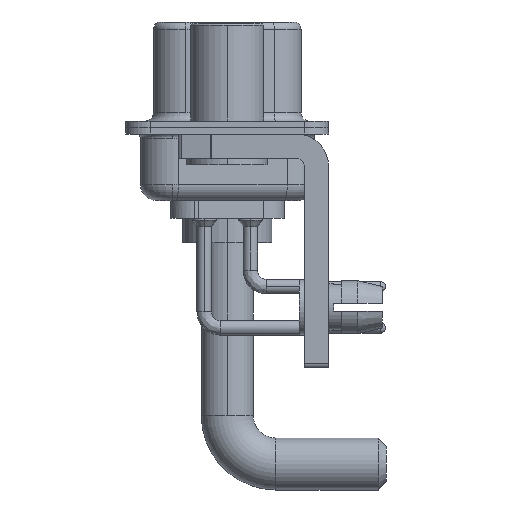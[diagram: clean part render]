
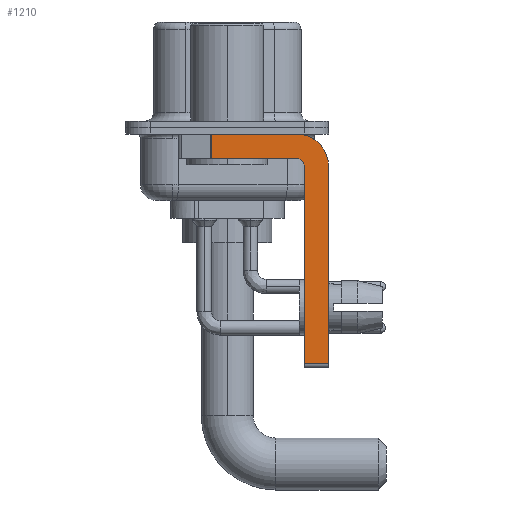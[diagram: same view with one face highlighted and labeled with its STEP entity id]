
A CAD part, left-side view. The second image highlights one B-rep face of the part: STEP entity #1210.
In plain terms, the highlighted planar face has unit normal (-1, 0, 0).
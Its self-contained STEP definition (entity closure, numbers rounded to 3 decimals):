
#480 = EDGE_LOOP ( 'NONE', ( #19807, #501, #16413, #14177, #4503, #20242, #6594, #23680 ) ) ;
#501 = ORIENTED_EDGE ( 'NONE', *, *, #6013, .T. ) ;
#781 = CARTESIAN_POINT ( 'NONE',  ( -2.9, -4.25, -0.4 ) ) ;
#921 = VERTEX_POINT ( 'NONE', #22389 ) ;
#944 = DIRECTION ( 'NONE',  ( 0., 0., -1. ) ) ;
#1027 = LINE ( 'NONE', #12141, #16594 ) ;
#1210 = ADVANCED_FACE ( 'NONE', ( #3372 ), #12655, .F. ) ;
#1835 = CARTESIAN_POINT ( 'NONE',  ( -2.9, -4.25, -2.4 ) ) ;
#1928 = DIRECTION ( 'NONE',  ( 0., -1., 0. ) ) ;
#2697 = DIRECTION ( 'NONE',  ( 0., 0., 1. ) ) ;
#3012 = CARTESIAN_POINT ( 'NONE',  ( -2.9, -4.25, -2.4 ) ) ;
#3253 = VERTEX_POINT ( 'NONE', #24991 ) ;
#3372 = FACE_OUTER_BOUND ( 'NONE', #480, .T. ) ;
#3839 = CARTESIAN_POINT ( 'NONE',  ( -2.9, -6.25, -2.4 ) ) ;
#4288 = CIRCLE ( 'NONE', #28021, 2. ) ;
#4343 = CARTESIAN_POINT ( 'NONE',  ( -2.9, -4.25, -14.55 ) ) ;
#4503 = ORIENTED_EDGE ( 'NONE', *, *, #25401, .F. ) ;
#4635 = LINE ( 'NONE', #4343, #18457 ) ;
#5493 = DIRECTION ( 'NONE',  ( 1., 0., 0. ) ) ;
#5538 = LINE ( 'NONE', #7837, #13043 ) ;
#5593 = VERTEX_POINT ( 'NONE', #27195 ) ;
#5756 = VECTOR ( 'NONE', #2697, 1000. ) ;
#6013 = EDGE_CURVE ( 'NONE', #3253, #921, #9756, .T. ) ;
#6594 = ORIENTED_EDGE ( 'NONE', *, *, #28598, .F. ) ;
#6961 = LINE ( 'NONE', #25174, #5756 ) ;
#7043 = VECTOR ( 'NONE', #12027, 1000. ) ;
#7492 = VERTEX_POINT ( 'NONE', #781 ) ;
#7837 = CARTESIAN_POINT ( 'NONE',  ( -2.9, 3., -0.4 ) ) ;
#8953 = CARTESIAN_POINT ( 'NONE',  ( -2.9, -4.25, -1.9 ) ) ;
#9756 = LINE ( 'NONE', #14622, #7043 ) ;
#11000 = CARTESIAN_POINT ( 'NONE',  ( -2.9, -4.75, -14.55 ) ) ;
#12027 = DIRECTION ( 'NONE',  ( 0., 0., -1. ) ) ;
#12141 = CARTESIAN_POINT ( 'NONE',  ( -2.9, -6.25, -2.4 ) ) ;
#12408 = CARTESIAN_POINT ( 'NONE',  ( -2.9, -4.25, -1.9 ) ) ;
#12599 = DIRECTION ( 'NONE',  ( -1., 0., 0. ) ) ;
#12655 = PLANE ( 'NONE',  #13497 ) ;
#12913 = VERTEX_POINT ( 'NONE', #11000 ) ;
#12959 = DIRECTION ( 'NONE',  ( 0., 0., -1. ) ) ;
#13043 = VECTOR ( 'NONE', #17099, 1000. ) ;
#13497 = AXIS2_PLACEMENT_3D ( 'NONE', #1835, #29456, #12959 ) ;
#14177 = ORIENTED_EDGE ( 'NONE', *, *, #24226, .F. ) ;
#14622 = CARTESIAN_POINT ( 'NONE',  ( -2.9, 0.978, -1.9 ) ) ;
#15515 = DIRECTION ( 'NONE',  ( 0., 1., 0. ) ) ;
#16413 = ORIENTED_EDGE ( 'NONE', *, *, #25262, .F. ) ;
#16594 = VECTOR ( 'NONE', #21378, 1000. ) ;
#16949 = AXIS2_PLACEMENT_3D ( 'NONE', #3012, #12599, #26365 ) ;
#17099 = DIRECTION ( 'NONE',  ( 0., -1., 0. ) ) ;
#18457 = VECTOR ( 'NONE', #1928, 1000. ) ;
#19239 = VERTEX_POINT ( 'NONE', #12408 ) ;
#19807 = ORIENTED_EDGE ( 'NONE', *, *, #24771, .F. ) ;
#20242 = ORIENTED_EDGE ( 'NONE', *, *, #27013, .T. ) ;
#20532 = VERTEX_POINT ( 'NONE', #24381 ) ;
#21378 = DIRECTION ( 'NONE',  ( 0., 0., -1. ) ) ;
#22046 = CARTESIAN_POINT ( 'NONE',  ( -2.9, -4.25, -2.4 ) ) ;
#22176 = LINE ( 'NONE', #8953, #26571 ) ;
#22389 = CARTESIAN_POINT ( 'NONE',  ( -2.9, 0.978, -1.9 ) ) ;
#23332 = EDGE_CURVE ( 'NONE', #7492, #23453, #4288, .T. ) ;
#23453 = VERTEX_POINT ( 'NONE', #3839 ) ;
#23680 = ORIENTED_EDGE ( 'NONE', *, *, #23332, .F. ) ;
#24226 = EDGE_CURVE ( 'NONE', #20532, #19239, #24692, .T. ) ;
#24381 = CARTESIAN_POINT ( 'NONE',  ( -2.9, -4.75, -2.4 ) ) ;
#24692 = CIRCLE ( 'NONE', #16949, 0.5 ) ;
#24771 = EDGE_CURVE ( 'NONE', #3253, #7492, #5538, .T. ) ;
#24991 = CARTESIAN_POINT ( 'NONE',  ( -2.9, 0.978, -0.4 ) ) ;
#25174 = CARTESIAN_POINT ( 'NONE',  ( -2.9, -4.75, -14.8 ) ) ;
#25262 = EDGE_CURVE ( 'NONE', #19239, #921, #22176, .T. ) ;
#25401 = EDGE_CURVE ( 'NONE', #12913, #20532, #6961, .T. ) ;
#26365 = DIRECTION ( 'NONE',  ( 0., 0., 1. ) ) ;
#26571 = VECTOR ( 'NONE', #15515, 1000. ) ;
#27013 = EDGE_CURVE ( 'NONE', #12913, #5593, #4635, .T. ) ;
#27195 = CARTESIAN_POINT ( 'NONE',  ( -2.9, -6.25, -14.55 ) ) ;
#28021 = AXIS2_PLACEMENT_3D ( 'NONE', #22046, #5493, #944 ) ;
#28598 = EDGE_CURVE ( 'NONE', #23453, #5593, #1027, .T. ) ;
#29456 = DIRECTION ( 'NONE',  ( 1., 0., 0. ) ) ;
